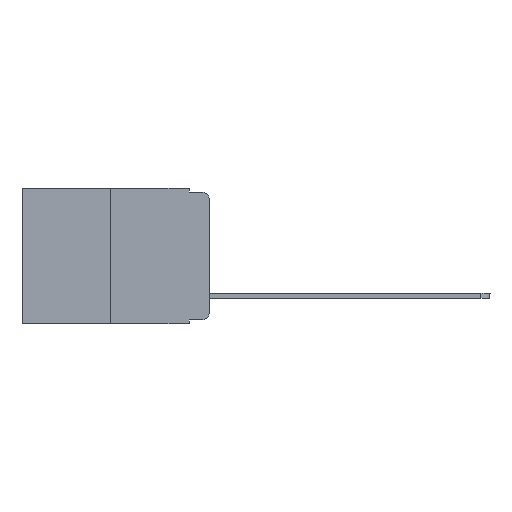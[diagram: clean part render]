
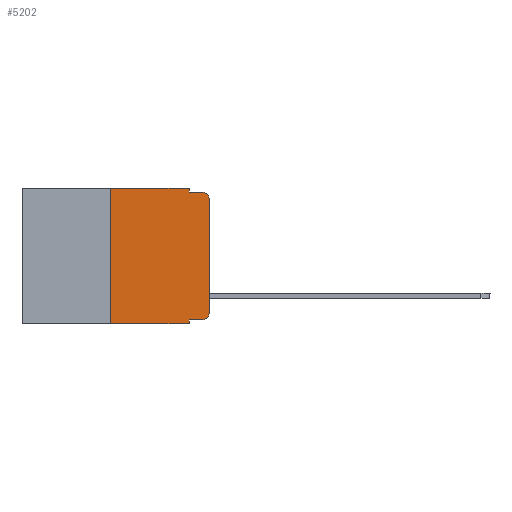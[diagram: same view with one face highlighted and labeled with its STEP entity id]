
A CAD part, left-side view. The second image highlights one B-rep face of the part: STEP entity #5202.
In plain terms, the highlighted planar face has unit normal (-1, 0, 0).
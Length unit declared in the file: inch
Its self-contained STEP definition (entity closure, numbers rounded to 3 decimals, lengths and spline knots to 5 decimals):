
#177 = VERTEX_POINT ( 'NONE', #6090 ) ;
#361 = CARTESIAN_POINT ( 'NONE',  ( 0., 0.473, 0. ) ) ;
#584 = LINE ( 'NONE', #3895, #8009 ) ;
#695 = CARTESIAN_POINT ( 'NONE',  ( 0., 0.25, 0. ) ) ;
#736 = VERTEX_POINT ( 'NONE', #8127 ) ;
#800 = AXIS2_PLACEMENT_3D ( 'NONE', #4210, #11267, #5942 ) ;
#964 = LINE ( 'NONE', #695, #3012 ) ;
#1007 = VERTEX_POINT ( 'NONE', #3515 ) ;
#1037 = FACE_OUTER_BOUND ( 'NONE', #7206, .T. ) ;
#1280 = LINE ( 'NONE', #1587, #10373 ) ;
#1418 = LINE ( 'NONE', #4043, #8579 ) ;
#1560 = DIRECTION ( 'NONE',  ( 0., -1., 0. ) ) ;
#1587 = CARTESIAN_POINT ( 'NONE',  ( 0., 0.051, -0.333 ) ) ;
#1670 = CARTESIAN_POINT ( 'NONE',  ( 0., 0.051, 0. ) ) ;
#1899 = DIRECTION ( 'NONE',  ( -1., 0., 0. ) ) ;
#1904 = VERTEX_POINT ( 'NONE', #10390 ) ;
#2006 = EDGE_CURVE ( 'NONE', #7078, #1904, #6717, .T. ) ;
#2256 = ORIENTED_EDGE ( 'NONE', *, *, #8455, .F. ) ;
#2389 = AXIS2_PLACEMENT_3D ( 'NONE', #10667, #1899, #4453 ) ;
#2499 = VERTEX_POINT ( 'NONE', #4974 ) ;
#2673 = CARTESIAN_POINT ( 'NONE',  ( 0., 0.051, -0.01 ) ) ;
#2709 = VERTEX_POINT ( 'NONE', #2817 ) ;
#2817 = CARTESIAN_POINT ( 'NONE',  ( 0., 0.02, -0.01 ) ) ;
#2943 = PLANE ( 'NONE',  #10714 ) ;
#2961 = EDGE_CURVE ( 'NONE', #8176, #2709, #5540, .T. ) ;
#3012 = VECTOR ( 'NONE', #5109, 39.37008 ) ;
#3035 = CIRCLE ( 'NONE', #2389, 0.02 ) ;
#3504 = ORIENTED_EDGE ( 'NONE', *, *, #2006, .T. ) ;
#3515 = CARTESIAN_POINT ( 'NONE',  ( 0., 0.25, 0. ) ) ;
#3651 = EDGE_CURVE ( 'NONE', #736, #7754, #1280, .T. ) ;
#3895 = CARTESIAN_POINT ( 'NONE',  ( 0., 0., 0. ) ) ;
#3993 = DIRECTION ( 'NONE',  ( 0., 0., -1. ) ) ;
#4027 = LINE ( 'NONE', #7357, #5643 ) ;
#4043 = CARTESIAN_POINT ( 'NONE',  ( 0., 0.051, 0. ) ) ;
#4196 = EDGE_CURVE ( 'NONE', #736, #1904, #1418, .T. ) ;
#4210 = CARTESIAN_POINT ( 'NONE',  ( 0., 0.02, -0.03 ) ) ;
#4453 = DIRECTION ( 'NONE',  ( 0., 0., -1. ) ) ;
#4589 = EDGE_CURVE ( 'NONE', #177, #8176, #584, .T. ) ;
#4666 = ORIENTED_EDGE ( 'NONE', *, *, #3651, .T. ) ;
#4799 = DIRECTION ( 'NONE',  ( 0., 0., -1. ) ) ;
#4891 = LINE ( 'NONE', #2673, #6792 ) ;
#4974 = CARTESIAN_POINT ( 'NONE',  ( 0., 0.051, -0.01 ) ) ;
#5098 = EDGE_CURVE ( 'NONE', #2499, #2709, #4891, .T. ) ;
#5109 = DIRECTION ( 'NONE',  ( 0., 0., 1. ) ) ;
#5123 = CARTESIAN_POINT ( 'NONE',  ( 0., 0.473, 0. ) ) ;
#5202 = ADVANCED_FACE ( 'NONE', ( #1037 ), #2943, .F. ) ;
#5540 = CIRCLE ( 'NONE', #800, 0.02 ) ;
#5643 = VECTOR ( 'NONE', #4799, 39.37008 ) ;
#5666 = ORIENTED_EDGE ( 'NONE', *, *, #2961, .T. ) ;
#5812 = ORIENTED_EDGE ( 'NONE', *, *, #4196, .F. ) ;
#5942 = DIRECTION ( 'NONE',  ( 0., 0., -1. ) ) ;
#5971 = ORIENTED_EDGE ( 'NONE', *, *, #5098, .F. ) ;
#6090 = CARTESIAN_POINT ( 'NONE',  ( 0., 0., -0.313 ) ) ;
#6357 = VERTEX_POINT ( 'NONE', #1670 ) ;
#6717 = LINE ( 'NONE', #7031, #11044 ) ;
#6792 = VECTOR ( 'NONE', #7267, 39.37008 ) ;
#7031 = CARTESIAN_POINT ( 'NONE',  ( 0., 0.473, -0.343 ) ) ;
#7078 = VERTEX_POINT ( 'NONE', #10374 ) ;
#7206 = EDGE_LOOP ( 'NONE', ( #9883, #5666, #5971, #8810, #2256, #10377, #3504, #5812, #4666, #9579 ) ) ;
#7267 = DIRECTION ( 'NONE',  ( 0., -1., 0. ) ) ;
#7357 = CARTESIAN_POINT ( 'NONE',  ( 0., 0.051, 0. ) ) ;
#7569 = DIRECTION ( 'NONE',  ( 0., 0., -1. ) ) ;
#7630 = DIRECTION ( 'NONE',  ( 0., -1., 0. ) ) ;
#7754 = VERTEX_POINT ( 'NONE', #9220 ) ;
#7902 = DIRECTION ( 'NONE',  ( 0., -1., 0. ) ) ;
#8009 = VECTOR ( 'NONE', #9984, 39.37008 ) ;
#8078 = EDGE_CURVE ( 'NONE', #7754, #177, #3035, .T. ) ;
#8127 = CARTESIAN_POINT ( 'NONE',  ( 0., 0.051, -0.333 ) ) ;
#8176 = VERTEX_POINT ( 'NONE', #10888 ) ;
#8266 = VECTOR ( 'NONE', #1560, 39.37008 ) ;
#8455 = EDGE_CURVE ( 'NONE', #1007, #6357, #10617, .T. ) ;
#8579 = VECTOR ( 'NONE', #7569, 39.37008 ) ;
#8810 = ORIENTED_EDGE ( 'NONE', *, *, #9022, .F. ) ;
#9022 = EDGE_CURVE ( 'NONE', #6357, #2499, #4027, .T. ) ;
#9204 = DIRECTION ( 'NONE',  ( 1., 0., 0. ) ) ;
#9220 = CARTESIAN_POINT ( 'NONE',  ( 0., 0.02, -0.333 ) ) ;
#9579 = ORIENTED_EDGE ( 'NONE', *, *, #8078, .T. ) ;
#9883 = ORIENTED_EDGE ( 'NONE', *, *, #4589, .T. ) ;
#9919 = EDGE_CURVE ( 'NONE', #7078, #1007, #964, .T. ) ;
#9984 = DIRECTION ( 'NONE',  ( 0., 0., 1. ) ) ;
#10373 = VECTOR ( 'NONE', #7630, 39.37008 ) ;
#10374 = CARTESIAN_POINT ( 'NONE',  ( 0., 0.25, -0.343 ) ) ;
#10377 = ORIENTED_EDGE ( 'NONE', *, *, #9919, .F. ) ;
#10390 = CARTESIAN_POINT ( 'NONE',  ( 0., 0.051, -0.343 ) ) ;
#10617 = LINE ( 'NONE', #5123, #8266 ) ;
#10667 = CARTESIAN_POINT ( 'NONE',  ( 0., 0.02, -0.313 ) ) ;
#10714 = AXIS2_PLACEMENT_3D ( 'NONE', #361, #9204, #3993 ) ;
#10888 = CARTESIAN_POINT ( 'NONE',  ( 0., 0., -0.03 ) ) ;
#11044 = VECTOR ( 'NONE', #7902, 39.37008 ) ;
#11267 = DIRECTION ( 'NONE',  ( -1., 0., 0. ) ) ;
